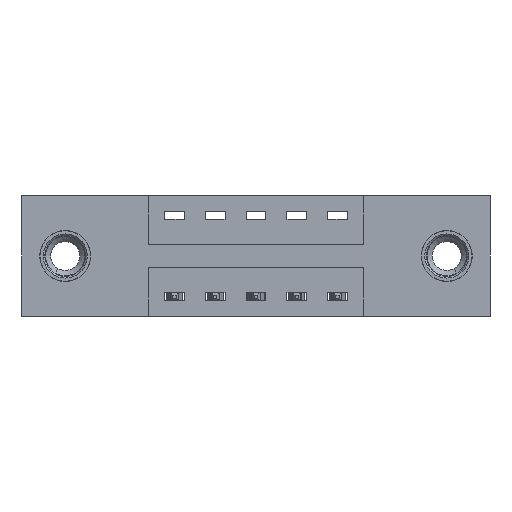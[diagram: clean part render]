
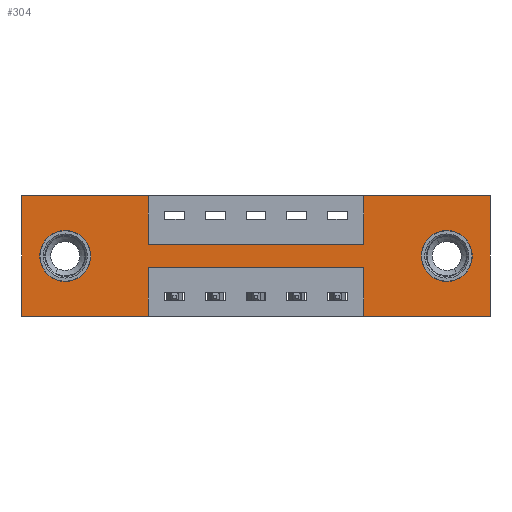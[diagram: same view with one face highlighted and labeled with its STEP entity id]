
A CAD part, front view. The second image highlights one B-rep face of the part: STEP entity #304.
In plain terms, the highlighted planar face has unit normal (0, -1, 0).
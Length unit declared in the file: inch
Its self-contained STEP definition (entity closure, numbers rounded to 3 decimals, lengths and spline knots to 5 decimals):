
#89 = AXIS2_PLACEMENT_3D ( 'NONE', #898, #8824, #3818 ) ;
#304 = ADVANCED_FACE ( 'NONE', ( #7113, #8165, #10183 ), #12387, .T. ) ;
#314 = ORIENTED_EDGE ( 'NONE', *, *, #12522, .F. ) ;
#525 = CARTESIAN_POINT ( 'NONE',  ( 0.1325, 0., -0.263 ) ) ;
#672 = VECTOR ( 'NONE', #11125, 39.37008 ) ;
#727 = DIRECTION ( 'NONE',  ( -1., 0., 0. ) ) ;
#732 = EDGE_CURVE ( 'NONE', #12229, #8031, #5681, .T. ) ;
#898 = CARTESIAN_POINT ( 'NONE',  ( 0.1325, 0., -0.185 ) ) ;
#930 = VERTEX_POINT ( 'NONE', #1733 ) ;
#949 = VERTEX_POINT ( 'NONE', #11661 ) ;
#1023 = ORIENTED_EDGE ( 'NONE', *, *, #10701, .F. ) ;
#1149 = EDGE_CURVE ( 'NONE', #930, #8829, #11858, .T. ) ;
#1284 = LINE ( 'NONE', #7893, #12166 ) ;
#1478 = ORIENTED_EDGE ( 'NONE', *, *, #12630, .F. ) ;
#1733 = CARTESIAN_POINT ( 'NONE',  ( 0.3875, 0., -0.15 ) ) ;
#1824 = CARTESIAN_POINT ( 'NONE',  ( 1.435, 0., -0.37 ) ) ;
#2039 = ORIENTED_EDGE ( 'NONE', *, *, #1149, .F. ) ;
#2125 = CARTESIAN_POINT ( 'NONE',  ( 1.0475, 0., 0. ) ) ;
#2208 = VECTOR ( 'NONE', #4074, 39.37008 ) ;
#2460 = DIRECTION ( 'NONE',  ( 0., 0., -1. ) ) ;
#2524 = VECTOR ( 'NONE', #5586, 39.37008 ) ;
#2536 = CARTESIAN_POINT ( 'NONE',  ( 1.435, 0., 0. ) ) ;
#2675 = ORIENTED_EDGE ( 'NONE', *, *, #5306, .F. ) ;
#2853 = CARTESIAN_POINT ( 'NONE',  ( 1.435, 0., 0. ) ) ;
#2961 = DIRECTION ( 'NONE',  ( 1., 0., 0. ) ) ;
#3008 = ORIENTED_EDGE ( 'NONE', *, *, #10045, .T. ) ;
#3030 = CARTESIAN_POINT ( 'NONE',  ( 0., 0., 0. ) ) ;
#3154 = VECTOR ( 'NONE', #3443, 39.37008 ) ;
#3187 = AXIS2_PLACEMENT_3D ( 'NONE', #6454, #8417, #2460 ) ;
#3228 = VERTEX_POINT ( 'NONE', #7070 ) ;
#3324 = LINE ( 'NONE', #12063, #2208 ) ;
#3413 = CARTESIAN_POINT ( 'NONE',  ( 0.3875, 0., -0.15 ) ) ;
#3422 = EDGE_CURVE ( 'NONE', #4082, #9118, #9204, .T. ) ;
#3443 = DIRECTION ( 'NONE',  ( 0., 0., 1. ) ) ;
#3647 = CARTESIAN_POINT ( 'NONE',  ( 0.3875, 0., -0.22 ) ) ;
#3655 = VERTEX_POINT ( 'NONE', #12117 ) ;
#3703 = ORIENTED_EDGE ( 'NONE', *, *, #8151, .F. ) ;
#3745 = DIRECTION ( 'NONE',  ( 1., 0., 0. ) ) ;
#3784 = DIRECTION ( 'NONE',  ( 0., 1., 0. ) ) ;
#3793 = VERTEX_POINT ( 'NONE', #2125 ) ;
#3818 = DIRECTION ( 'NONE',  ( 0., 0., 1. ) ) ;
#3899 = CIRCLE ( 'NONE', #5948, 0.078 ) ;
#4074 = DIRECTION ( 'NONE',  ( -1., 0., 0. ) ) ;
#4082 = VERTEX_POINT ( 'NONE', #6055 ) ;
#4179 = CARTESIAN_POINT ( 'NONE',  ( 1.0475, 0., -0.37 ) ) ;
#4573 = CARTESIAN_POINT ( 'NONE',  ( 1.0475, 0., 0. ) ) ;
#4575 = VERTEX_POINT ( 'NONE', #12576 ) ;
#4930 = VECTOR ( 'NONE', #727, 39.37008 ) ;
#4948 = EDGE_LOOP ( 'NONE', ( #8204, #3008 ) ) ;
#4963 = ORIENTED_EDGE ( 'NONE', *, *, #12873, .F. ) ;
#5180 = ORIENTED_EDGE ( 'NONE', *, *, #732, .F. ) ;
#5306 = EDGE_CURVE ( 'NONE', #3793, #12229, #12516, .T. ) ;
#5367 = LINE ( 'NONE', #4573, #2524 ) ;
#5461 = DIRECTION ( 'NONE',  ( 1., 0., 0. ) ) ;
#5586 = DIRECTION ( 'NONE',  ( 0., 0., 1. ) ) ;
#5681 = LINE ( 'NONE', #2536, #12182 ) ;
#5871 = EDGE_CURVE ( 'NONE', #8031, #10911, #3324, .T. ) ;
#5948 = AXIS2_PLACEMENT_3D ( 'NONE', #12734, #3784, #10845 ) ;
#6055 = CARTESIAN_POINT ( 'NONE',  ( 0., 0., -0.37 ) ) ;
#6454 = CARTESIAN_POINT ( 'NONE',  ( 0., 0., -0.37 ) ) ;
#6616 = CARTESIAN_POINT ( 'NONE',  ( 0.3875, 0., -0.37 ) ) ;
#6884 = ORIENTED_EDGE ( 'NONE', *, *, #3422, .F. ) ;
#6896 = EDGE_CURVE ( 'NONE', #3655, #11851, #7330, .T. ) ;
#6899 = DIRECTION ( 'NONE',  ( 0., 0., -1. ) ) ;
#6986 = DIRECTION ( 'NONE',  ( 0., 0., -1. ) ) ;
#6995 = CARTESIAN_POINT ( 'NONE',  ( 1.0475, 0., -0.37 ) ) ;
#7070 = CARTESIAN_POINT ( 'NONE',  ( 0.3875, 0., -0.22 ) ) ;
#7112 = VERTEX_POINT ( 'NONE', #11438 ) ;
#7113 = FACE_BOUND ( 'NONE', #12574, .T. ) ;
#7126 = CARTESIAN_POINT ( 'NONE',  ( 1.3025, 0., -0.107 ) ) ;
#7330 = CIRCLE ( 'NONE', #7397, 0.078 ) ;
#7397 = AXIS2_PLACEMENT_3D ( 'NONE', #9952, #9763, #6986 ) ;
#7469 = EDGE_CURVE ( 'NONE', #4575, #4082, #8342, .T. ) ;
#7563 = CARTESIAN_POINT ( 'NONE',  ( 0.1325, 0., -0.107 ) ) ;
#7599 = CARTESIAN_POINT ( 'NONE',  ( 0., 0., -0.37 ) ) ;
#7664 = AXIS2_PLACEMENT_3D ( 'NONE', #10989, #12009, #12091 ) ;
#7709 = ORIENTED_EDGE ( 'NONE', *, *, #9886, .T. ) ;
#7792 = CARTESIAN_POINT ( 'NONE',  ( 0., 0., 0. ) ) ;
#7893 = CARTESIAN_POINT ( 'NONE',  ( 0., 0., 0. ) ) ;
#7926 = EDGE_CURVE ( 'NONE', #11135, #10757, #12685, .T. ) ;
#7995 = EDGE_LOOP ( 'NONE', ( #12499, #1023, #4963, #11999, #5180, #2675, #314, #2039, #3703, #1478, #6884, #10784 ) ) ;
#8031 = VERTEX_POINT ( 'NONE', #1824 ) ;
#8151 = EDGE_CURVE ( 'NONE', #949, #930, #9737, .T. ) ;
#8165 = FACE_BOUND ( 'NONE', #4948, .T. ) ;
#8204 = ORIENTED_EDGE ( 'NONE', *, *, #7926, .T. ) ;
#8342 = LINE ( 'NONE', #7599, #8622 ) ;
#8417 = DIRECTION ( 'NONE',  ( 0., -1., 0. ) ) ;
#8622 = VECTOR ( 'NONE', #10756, 39.37008 ) ;
#8824 = DIRECTION ( 'NONE',  ( 0., 1., 0. ) ) ;
#8829 = VERTEX_POINT ( 'NONE', #9934 ) ;
#8977 = VECTOR ( 'NONE', #6899, 39.37008 ) ;
#9008 = CIRCLE ( 'NONE', #7664, 0.078 ) ;
#9118 = VERTEX_POINT ( 'NONE', #7792 ) ;
#9168 = VECTOR ( 'NONE', #3745, 39.37008 ) ;
#9204 = LINE ( 'NONE', #10205, #672 ) ;
#9454 = DIRECTION ( 'NONE',  ( 0., 0., -1. ) ) ;
#9720 = LINE ( 'NONE', #6616, #12101 ) ;
#9737 = LINE ( 'NONE', #12716, #8977 ) ;
#9763 = DIRECTION ( 'NONE',  ( 0., 1., 0. ) ) ;
#9886 = EDGE_CURVE ( 'NONE', #11851, #3655, #3899, .T. ) ;
#9934 = CARTESIAN_POINT ( 'NONE',  ( 1.0475, 0., -0.15 ) ) ;
#9952 = CARTESIAN_POINT ( 'NONE',  ( 1.3025, 0., -0.185 ) ) ;
#9969 = ORIENTED_EDGE ( 'NONE', *, *, #6896, .T. ) ;
#10045 = EDGE_CURVE ( 'NONE', #10757, #11135, #9008, .T. ) ;
#10183 = FACE_OUTER_BOUND ( 'NONE', #7995, .T. ) ;
#10205 = CARTESIAN_POINT ( 'NONE',  ( 0., 0., 0. ) ) ;
#10327 = VECTOR ( 'NONE', #5461, 39.37008 ) ;
#10506 = EDGE_CURVE ( 'NONE', #3228, #4575, #9720, .T. ) ;
#10701 = EDGE_CURVE ( 'NONE', #7112, #3228, #11301, .T. ) ;
#10756 = DIRECTION ( 'NONE',  ( -1., 0., 0. ) ) ;
#10757 = VERTEX_POINT ( 'NONE', #525 ) ;
#10784 = ORIENTED_EDGE ( 'NONE', *, *, #7469, .F. ) ;
#10845 = DIRECTION ( 'NONE',  ( 0., 0., -1. ) ) ;
#10911 = VERTEX_POINT ( 'NONE', #6995 ) ;
#10989 = CARTESIAN_POINT ( 'NONE',  ( 0.1325, 0., -0.185 ) ) ;
#11125 = DIRECTION ( 'NONE',  ( 0., 0., 1. ) ) ;
#11135 = VERTEX_POINT ( 'NONE', #7563 ) ;
#11301 = LINE ( 'NONE', #3647, #4930 ) ;
#11438 = CARTESIAN_POINT ( 'NONE',  ( 1.0475, 0., -0.22 ) ) ;
#11661 = CARTESIAN_POINT ( 'NONE',  ( 0.3875, 0., 0. ) ) ;
#11851 = VERTEX_POINT ( 'NONE', #7126 ) ;
#11858 = LINE ( 'NONE', #3413, #9168 ) ;
#11999 = ORIENTED_EDGE ( 'NONE', *, *, #5871, .F. ) ;
#12009 = DIRECTION ( 'NONE',  ( 0., 1., 0. ) ) ;
#12024 = LINE ( 'NONE', #4179, #3154 ) ;
#12063 = CARTESIAN_POINT ( 'NONE',  ( 0., 0., -0.37 ) ) ;
#12091 = DIRECTION ( 'NONE',  ( 0., 0., 1. ) ) ;
#12101 = VECTOR ( 'NONE', #9454, 39.37008 ) ;
#12117 = CARTESIAN_POINT ( 'NONE',  ( 1.3025, 0., -0.263 ) ) ;
#12166 = VECTOR ( 'NONE', #2961, 39.37008 ) ;
#12182 = VECTOR ( 'NONE', #12415, 39.37008 ) ;
#12229 = VERTEX_POINT ( 'NONE', #2853 ) ;
#12387 = PLANE ( 'NONE',  #3187 ) ;
#12415 = DIRECTION ( 'NONE',  ( 0., 0., -1. ) ) ;
#12499 = ORIENTED_EDGE ( 'NONE', *, *, #10506, .F. ) ;
#12516 = LINE ( 'NONE', #3030, #10327 ) ;
#12522 = EDGE_CURVE ( 'NONE', #8829, #3793, #5367, .T. ) ;
#12574 = EDGE_LOOP ( 'NONE', ( #7709, #9969 ) ) ;
#12576 = CARTESIAN_POINT ( 'NONE',  ( 0.3875, 0., -0.37 ) ) ;
#12630 = EDGE_CURVE ( 'NONE', #9118, #949, #1284, .T. ) ;
#12685 = CIRCLE ( 'NONE', #89, 0.078 ) ;
#12716 = CARTESIAN_POINT ( 'NONE',  ( 0.3875, 0., 0. ) ) ;
#12734 = CARTESIAN_POINT ( 'NONE',  ( 1.3025, 0., -0.185 ) ) ;
#12873 = EDGE_CURVE ( 'NONE', #10911, #7112, #12024, .T. ) ;
